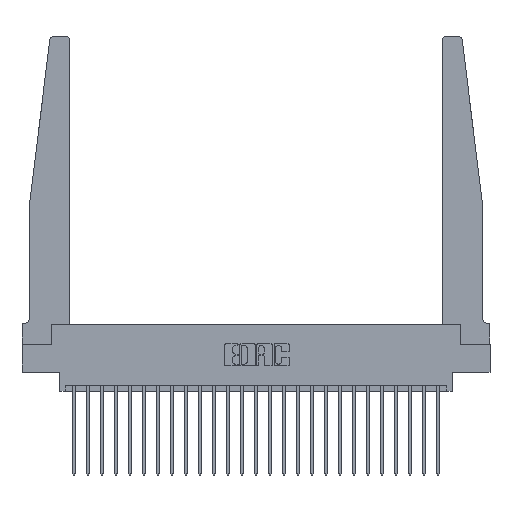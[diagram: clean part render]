
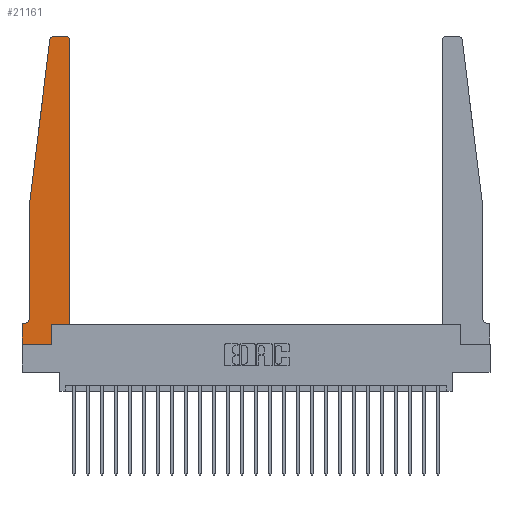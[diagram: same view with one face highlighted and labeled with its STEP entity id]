
A CAD part, top view. The second image highlights one B-rep face of the part: STEP entity #21161.
In plain terms, the highlighted planar face has unit normal (0, 0, 1).
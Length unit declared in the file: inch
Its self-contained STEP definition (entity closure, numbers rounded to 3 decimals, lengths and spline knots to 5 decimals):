
#309 = VERTEX_POINT ( 'NONE', #23931 ) ;
#490 = DIRECTION ( 'NONE',  ( 0., 0., 1. ) ) ;
#723 = VERTEX_POINT ( 'NONE', #19693 ) ;
#798 = ORIENTED_EDGE ( 'NONE', *, *, #18330, .T. ) ;
#855 = DIRECTION ( 'NONE',  ( 1., 0., 0. ) ) ;
#2100 = VERTEX_POINT ( 'NONE', #12618 ) ;
#2314 = VECTOR ( 'NONE', #23831, 39.37008 ) ;
#2631 = CIRCLE ( 'NONE', #20261, 0.03 ) ;
#2898 = LINE ( 'NONE', #10508, #2314 ) ;
#2968 = CARTESIAN_POINT ( 'NONE',  ( 0.425, 0.18, 0.37 ) ) ;
#2986 = CIRCLE ( 'NONE', #9988, 0.03 ) ;
#3304 = VERTEX_POINT ( 'NONE', #2968 ) ;
#3427 = ORIENTED_EDGE ( 'NONE', *, *, #15450, .T. ) ;
#3455 = CARTESIAN_POINT ( 'NONE',  ( 0.24675, 2.72367, 0.37 ) ) ;
#3460 = VERTEX_POINT ( 'NONE', #3455 ) ;
#3467 = CARTESIAN_POINT ( 'NONE',  ( 0.27653, 2.72, 0.37 ) ) ;
#3739 = EDGE_CURVE ( 'NONE', #21719, #309, #5149, .T. ) ;
#4514 = DIRECTION ( 'NONE',  ( 0., -1., 0. ) ) ;
#4683 = EDGE_CURVE ( 'NONE', #23583, #21719, #8793, .T. ) ;
#4774 = ORIENTED_EDGE ( 'NONE', *, *, #17550, .T. ) ;
#5149 = LINE ( 'NONE', #6358, #19694 ) ;
#5381 = DIRECTION ( 'NONE',  ( 1., 0., 0. ) ) ;
#5470 = VECTOR ( 'NONE', #17676, 39.37008 ) ;
#5938 = CARTESIAN_POINT ( 'NONE',  ( 0.065, 1.25, 0.37 ) ) ;
#6139 = CARTESIAN_POINT ( 'NONE',  ( 0., 0.1875, 0.37 ) ) ;
#6358 = CARTESIAN_POINT ( 'NONE',  ( 0., 0., 0.37 ) ) ;
#6744 = LINE ( 'NONE', #10456, #16191 ) ;
#7306 = LINE ( 'NONE', #22799, #21291 ) ;
#7379 = CARTESIAN_POINT ( 'NONE',  ( 0.065, 0.2375, 0.37 ) ) ;
#7646 = ORIENTED_EDGE ( 'NONE', *, *, #21393, .T. ) ;
#7771 = VECTOR ( 'NONE', #855, 39.37008 ) ;
#8251 = CARTESIAN_POINT ( 'NONE',  ( 0.015, 0.2375, 0.37 ) ) ;
#8729 = VERTEX_POINT ( 'NONE', #5938 ) ;
#8793 = LINE ( 'NONE', #18733, #18306 ) ;
#9135 = CARTESIAN_POINT ( 'NONE',  ( 0.2605, 0., 0.37 ) ) ;
#9221 = VECTOR ( 'NONE', #23936, 39.37008 ) ;
#9261 = VERTEX_POINT ( 'NONE', #7379 ) ;
#9402 = AXIS2_PLACEMENT_3D ( 'NONE', #8251, #21566, #10123 ) ;
#9624 = AXIS2_PLACEMENT_3D ( 'NONE', #6139, #490, #13714 ) ;
#9749 = VERTEX_POINT ( 'NONE', #20162 ) ;
#9861 = ORIENTED_EDGE ( 'NONE', *, *, #3739, .T. ) ;
#9862 = EDGE_CURVE ( 'NONE', #723, #3460, #2986, .T. ) ;
#9988 = AXIS2_PLACEMENT_3D ( 'NONE', #3467, #16689, #5381 ) ;
#10123 = DIRECTION ( 'NONE',  ( -1., 0., 0. ) ) ;
#10425 = CARTESIAN_POINT ( 'NONE',  ( 0.395, 2.72, 0.37 ) ) ;
#10456 = CARTESIAN_POINT ( 'NONE',  ( 0.065, 1.25, 0.37 ) ) ;
#10463 = LINE ( 'NONE', #15762, #5470 ) ;
#10508 = CARTESIAN_POINT ( 'NONE',  ( 0.065, 1.25, 0.37 ) ) ;
#11379 = DIRECTION ( 'NONE',  ( 1., 0., 0. ) ) ;
#11651 = EDGE_CURVE ( 'NONE', #3304, #9749, #23766, .T. ) ;
#11972 = CARTESIAN_POINT ( 'NONE',  ( 0.2605, 0.18, 0.37 ) ) ;
#12021 = CIRCLE ( 'NONE', #9402, 0.05 ) ;
#12344 = DIRECTION ( 'NONE',  ( 1., 0., 0. ) ) ;
#12396 = CARTESIAN_POINT ( 'NONE',  ( 0.425, 0.18, 0.37 ) ) ;
#12419 = ORIENTED_EDGE ( 'NONE', *, *, #13958, .T. ) ;
#12618 = CARTESIAN_POINT ( 'NONE',  ( 0.395, 2.75, 0.37 ) ) ;
#12709 = ORIENTED_EDGE ( 'NONE', *, *, #4683, .T. ) ;
#12892 = ORIENTED_EDGE ( 'NONE', *, *, #9862, .T. ) ;
#12896 = EDGE_CURVE ( 'NONE', #9749, #2100, #2631, .T. ) ;
#13714 = DIRECTION ( 'NONE',  ( 1., 0., 0. ) ) ;
#13958 = EDGE_CURVE ( 'NONE', #309, #16948, #7306, .T. ) ;
#14177 = EDGE_CURVE ( 'NONE', #9261, #23583, #12021, .T. ) ;
#14480 = EDGE_LOOP ( 'NONE', ( #3427, #12892, #24027, #7646, #20359, #12709, #9861, #12419, #798, #4774, #19317, #19080 ) ) ;
#15450 = EDGE_CURVE ( 'NONE', #2100, #723, #10463, .T. ) ;
#15762 = CARTESIAN_POINT ( 'NONE',  ( 0.25, 2.75, 0.37 ) ) ;
#16191 = VECTOR ( 'NONE', #21901, 39.37008 ) ;
#16339 = CARTESIAN_POINT ( 'NONE',  ( 0.2605, 0.18, 0.37 ) ) ;
#16689 = DIRECTION ( 'NONE',  ( 0., 0., 1. ) ) ;
#16948 = VERTEX_POINT ( 'NONE', #9135 ) ;
#17550 = EDGE_CURVE ( 'NONE', #23223, #3304, #17840, .T. ) ;
#17676 = DIRECTION ( 'NONE',  ( -1., 0., 0. ) ) ;
#17840 = LINE ( 'NONE', #23571, #7771 ) ;
#18306 = VECTOR ( 'NONE', #20683, 39.37008 ) ;
#18330 = EDGE_CURVE ( 'NONE', #16948, #23223, #19368, .T. ) ;
#18733 = CARTESIAN_POINT ( 'NONE',  ( 0.065, 0.1875, 0.37 ) ) ;
#19080 = ORIENTED_EDGE ( 'NONE', *, *, #12896, .T. ) ;
#19317 = ORIENTED_EDGE ( 'NONE', *, *, #11651, .T. ) ;
#19322 = VECTOR ( 'NONE', #23797, 39.37008 ) ;
#19368 = LINE ( 'NONE', #16339, #9221 ) ;
#19693 = CARTESIAN_POINT ( 'NONE',  ( 0.27653, 2.75, 0.37 ) ) ;
#19694 = VECTOR ( 'NONE', #4514, 39.37008 ) ;
#20162 = CARTESIAN_POINT ( 'NONE',  ( 0.425, 2.72, 0.37 ) ) ;
#20261 = AXIS2_PLACEMENT_3D ( 'NONE', #10425, #23747, #12344 ) ;
#20359 = ORIENTED_EDGE ( 'NONE', *, *, #14177, .T. ) ;
#20443 = FACE_OUTER_BOUND ( 'NONE', #14480, .T. ) ;
#20560 = CARTESIAN_POINT ( 'NONE',  ( 0.015, 0.1875, 0.37 ) ) ;
#20683 = DIRECTION ( 'NONE',  ( -1., 0., 0. ) ) ;
#21139 = CARTESIAN_POINT ( 'NONE',  ( 0., 0.1875, 0.37 ) ) ;
#21161 = ADVANCED_FACE ( 'NONE', ( #20443 ), #23220, .T. ) ;
#21291 = VECTOR ( 'NONE', #11379, 39.37008 ) ;
#21393 = EDGE_CURVE ( 'NONE', #8729, #9261, #6744, .T. ) ;
#21566 = DIRECTION ( 'NONE',  ( 0., 0., -1. ) ) ;
#21719 = VERTEX_POINT ( 'NONE', #21139 ) ;
#21901 = DIRECTION ( 'NONE',  ( 0., -1., 0. ) ) ;
#22038 = EDGE_CURVE ( 'NONE', #3460, #8729, #2898, .T. ) ;
#22799 = CARTESIAN_POINT ( 'NONE',  ( 0., 0., 0.37 ) ) ;
#23220 = PLANE ( 'NONE',  #9624 ) ;
#23223 = VERTEX_POINT ( 'NONE', #11972 ) ;
#23571 = CARTESIAN_POINT ( 'NONE',  ( 0.425, 0.18, 0.37 ) ) ;
#23583 = VERTEX_POINT ( 'NONE', #20560 ) ;
#23747 = DIRECTION ( 'NONE',  ( 0., 0., 1. ) ) ;
#23766 = LINE ( 'NONE', #12396, #19322 ) ;
#23797 = DIRECTION ( 'NONE',  ( 0., 1., 0. ) ) ;
#23831 = DIRECTION ( 'NONE',  ( -0.122, -0.992, 0. ) ) ;
#23931 = CARTESIAN_POINT ( 'NONE',  ( 0., 0., 0.37 ) ) ;
#23936 = DIRECTION ( 'NONE',  ( 0., 1., 0. ) ) ;
#24027 = ORIENTED_EDGE ( 'NONE', *, *, #22038, .T. ) ;
